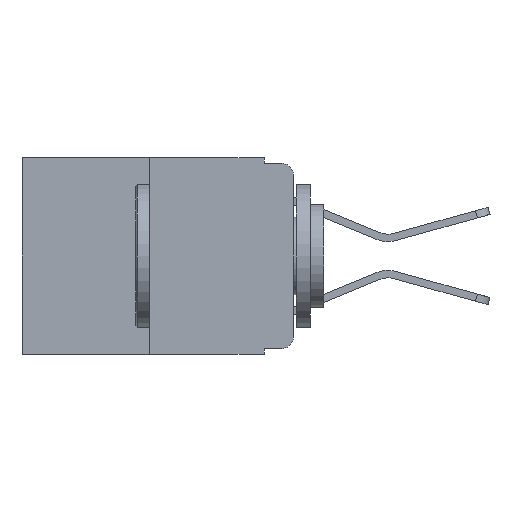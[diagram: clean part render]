
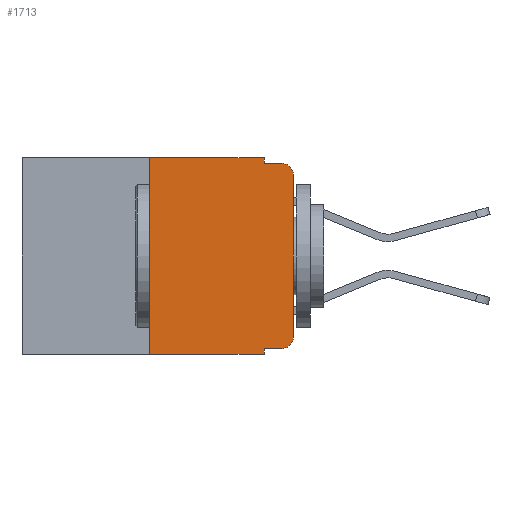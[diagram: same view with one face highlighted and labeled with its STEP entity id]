
A CAD part, left-side view. The second image highlights one B-rep face of the part: STEP entity #1713.
In plain terms, the highlighted planar face has unit normal (-1, 0, 0).
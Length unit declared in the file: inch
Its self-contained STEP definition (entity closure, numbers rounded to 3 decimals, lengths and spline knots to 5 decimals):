
#594 = VERTEX_POINT ( 'NONE', #3148 ) ;
#794 = CARTESIAN_POINT ( 'NONE',  ( 0., 0., 0. ) ) ;
#882 = VERTEX_POINT ( 'NONE', #5414 ) ;
#924 = ORIENTED_EDGE ( 'NONE', *, *, #8788, .T. ) ;
#1039 = DIRECTION ( 'NONE',  ( 0., -1., 0. ) ) ;
#1148 = VERTEX_POINT ( 'NONE', #8802 ) ;
#1444 = VECTOR ( 'NONE', #5822, 39.37008 ) ;
#1478 = ORIENTED_EDGE ( 'NONE', *, *, #3304, .F. ) ;
#1713 = ADVANCED_FACE ( 'NONE', ( #4669 ), #9364, .F. ) ;
#1726 = DIRECTION ( 'NONE',  ( -1., 0., 0. ) ) ;
#1748 = CARTESIAN_POINT ( 'NONE',  ( 0., 0.051, 0. ) ) ;
#1784 = EDGE_LOOP ( 'NONE', ( #924, #3475, #1478, #5923, #10101, #4225, #10578, #6692, #4753, #9001 ) ) ;
#2256 = EDGE_CURVE ( 'NONE', #10572, #594, #6094, .T. ) ;
#2352 = VECTOR ( 'NONE', #6412, 39.37008 ) ;
#2621 = EDGE_CURVE ( 'NONE', #882, #10572, #9687, .T. ) ;
#3148 = CARTESIAN_POINT ( 'NONE',  ( 0., 0.051, -0.01 ) ) ;
#3304 = EDGE_CURVE ( 'NONE', #594, #1148, #8571, .T. ) ;
#3354 = CIRCLE ( 'NONE', #3521, 0.02 ) ;
#3365 = CARTESIAN_POINT ( 'NONE',  ( 0., 0.473, -0.343 ) ) ;
#3431 = VERTEX_POINT ( 'NONE', #5684 ) ;
#3475 = ORIENTED_EDGE ( 'NONE', *, *, #7773, .T. ) ;
#3521 = AXIS2_PLACEMENT_3D ( 'NONE', #6087, #6083, #6075 ) ;
#3579 = DIRECTION ( 'NONE',  ( 0., -1., 0. ) ) ;
#3886 = VECTOR ( 'NONE', #7418, 39.37008 ) ;
#4225 = ORIENTED_EDGE ( 'NONE', *, *, #9155, .F. ) ;
#4368 = VECTOR ( 'NONE', #3579, 39.37008 ) ;
#4635 = LINE ( 'NONE', #3365, #4368 ) ;
#4669 = FACE_OUTER_BOUND ( 'NONE', #1784, .T. ) ;
#4753 = ORIENTED_EDGE ( 'NONE', *, *, #4888, .T. ) ;
#4799 = CARTESIAN_POINT ( 'NONE',  ( 0., 0., -0.313 ) ) ;
#4848 = CIRCLE ( 'NONE', #5200, 0.02 ) ;
#4861 = CARTESIAN_POINT ( 'NONE',  ( 0., 0.02, -0.333 ) ) ;
#4888 = EDGE_CURVE ( 'NONE', #7181, #5843, #10225, .T. ) ;
#5013 = DIRECTION ( 'NONE',  ( 0., -1., 0. ) ) ;
#5101 = CARTESIAN_POINT ( 'NONE',  ( 0., 0.473, 0. ) ) ;
#5103 = CARTESIAN_POINT ( 'NONE',  ( 0., 0.051, -0.333 ) ) ;
#5200 = AXIS2_PLACEMENT_3D ( 'NONE', #6714, #1726, #7518 ) ;
#5414 = CARTESIAN_POINT ( 'NONE',  ( 0., 0.25, 0. ) ) ;
#5555 = EDGE_CURVE ( 'NONE', #5969, #3431, #4635, .T. ) ;
#5629 = LINE ( 'NONE', #7156, #7521 ) ;
#5656 = EDGE_CURVE ( 'NONE', #5843, #5846, #3354, .T. ) ;
#5684 = CARTESIAN_POINT ( 'NONE',  ( 0., 0.051, -0.343 ) ) ;
#5762 = CARTESIAN_POINT ( 'NONE',  ( 0., 0.25, -0.343 ) ) ;
#5822 = DIRECTION ( 'NONE',  ( 0., 0., 1. ) ) ;
#5843 = VERTEX_POINT ( 'NONE', #4861 ) ;
#5846 = VERTEX_POINT ( 'NONE', #4799 ) ;
#5908 = CARTESIAN_POINT ( 'NONE',  ( 0., 0.473, 0. ) ) ;
#5923 = ORIENTED_EDGE ( 'NONE', *, *, #2256, .F. ) ;
#5969 = VERTEX_POINT ( 'NONE', #5762 ) ;
#5984 = CARTESIAN_POINT ( 'NONE',  ( 0., 0.051, 0. ) ) ;
#6071 = VECTOR ( 'NONE', #1039, 39.37008 ) ;
#6075 = DIRECTION ( 'NONE',  ( 0., 0., -1. ) ) ;
#6083 = DIRECTION ( 'NONE',  ( -1., 0., 0. ) ) ;
#6087 = CARTESIAN_POINT ( 'NONE',  ( 0., 0.02, -0.313 ) ) ;
#6094 = LINE ( 'NONE', #5984, #3886 ) ;
#6405 = VECTOR ( 'NONE', #9621, 39.37008 ) ;
#6412 = DIRECTION ( 'NONE',  ( 0., -1., 0. ) ) ;
#6658 = LINE ( 'NONE', #8827, #6405 ) ;
#6692 = ORIENTED_EDGE ( 'NONE', *, *, #7611, .F. ) ;
#6714 = CARTESIAN_POINT ( 'NONE',  ( 0., 0.02, -0.03 ) ) ;
#7134 = VECTOR ( 'NONE', #5013, 39.37008 ) ;
#7156 = CARTESIAN_POINT ( 'NONE',  ( 0., 0.25, 0. ) ) ;
#7181 = VERTEX_POINT ( 'NONE', #8308 ) ;
#7418 = DIRECTION ( 'NONE',  ( 0., 0., -1. ) ) ;
#7518 = DIRECTION ( 'NONE',  ( 0., 0., -1. ) ) ;
#7521 = VECTOR ( 'NONE', #10235, 39.37008 ) ;
#7611 = EDGE_CURVE ( 'NONE', #7181, #3431, #6658, .T. ) ;
#7773 = EDGE_CURVE ( 'NONE', #8129, #1148, #4848, .T. ) ;
#8129 = VERTEX_POINT ( 'NONE', #10245 ) ;
#8215 = CARTESIAN_POINT ( 'NONE',  ( 0., 0.051, -0.01 ) ) ;
#8267 = LINE ( 'NONE', #794, #1444 ) ;
#8308 = CARTESIAN_POINT ( 'NONE',  ( 0., 0.051, -0.333 ) ) ;
#8571 = LINE ( 'NONE', #8215, #2352 ) ;
#8788 = EDGE_CURVE ( 'NONE', #5846, #8129, #8267, .T. ) ;
#8802 = CARTESIAN_POINT ( 'NONE',  ( 0., 0.02, -0.01 ) ) ;
#8827 = CARTESIAN_POINT ( 'NONE',  ( 0., 0.051, 0. ) ) ;
#8872 = AXIS2_PLACEMENT_3D ( 'NONE', #5908, #10177, #9008 ) ;
#9001 = ORIENTED_EDGE ( 'NONE', *, *, #5656, .T. ) ;
#9008 = DIRECTION ( 'NONE',  ( 0., 0., -1. ) ) ;
#9155 = EDGE_CURVE ( 'NONE', #5969, #882, #5629, .T. ) ;
#9364 = PLANE ( 'NONE',  #8872 ) ;
#9621 = DIRECTION ( 'NONE',  ( 0., 0., -1. ) ) ;
#9687 = LINE ( 'NONE', #5101, #7134 ) ;
#10101 = ORIENTED_EDGE ( 'NONE', *, *, #2621, .F. ) ;
#10177 = DIRECTION ( 'NONE',  ( 1., 0., 0. ) ) ;
#10225 = LINE ( 'NONE', #5103, #6071 ) ;
#10235 = DIRECTION ( 'NONE',  ( 0., 0., 1. ) ) ;
#10245 = CARTESIAN_POINT ( 'NONE',  ( 0., 0., -0.03 ) ) ;
#10572 = VERTEX_POINT ( 'NONE', #1748 ) ;
#10578 = ORIENTED_EDGE ( 'NONE', *, *, #5555, .T. ) ;
